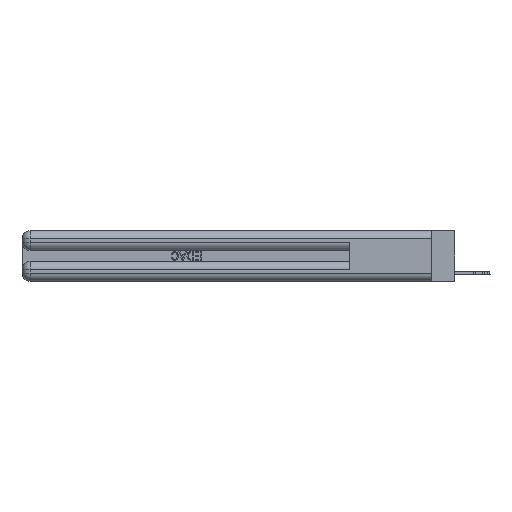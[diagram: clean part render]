
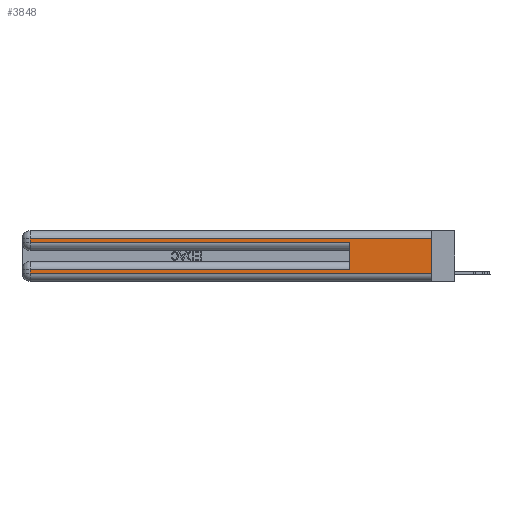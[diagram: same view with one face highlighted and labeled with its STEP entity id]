
A CAD part, left-side view. The second image highlights one B-rep face of the part: STEP entity #3848.
In plain terms, the highlighted planar face has unit normal (-1, 0, 0).
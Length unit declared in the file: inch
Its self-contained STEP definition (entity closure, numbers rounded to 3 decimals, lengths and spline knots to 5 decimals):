
#33 = VECTOR ( 'NONE', #11061, 39.37008 ) ;
#159 = EDGE_CURVE ( 'NONE', #11562, #15059, #29288, .T. ) ;
#877 = DIRECTION ( 'NONE',  ( 1., 0., 0. ) ) ;
#889 = CARTESIAN_POINT ( 'NONE',  ( 0., 0., 0.37 ) ) ;
#2600 = VERTEX_POINT ( 'NONE', #24273 ) ;
#3084 = LINE ( 'NONE', #10879, #33 ) ;
#3848 = ADVANCED_FACE ( 'NONE', ( #14192 ), #19877, .F. ) ;
#4034 = VECTOR ( 'NONE', #12437, 39.37008 ) ;
#4628 = CARTESIAN_POINT ( 'NONE',  ( 0., 0., 0.06 ) ) ;
#4669 = ORIENTED_EDGE ( 'NONE', *, *, #18117, .T. ) ;
#5305 = VECTOR ( 'NONE', #8779, 39.37008 ) ;
#5569 = VECTOR ( 'NONE', #26347, 39.37008 ) ;
#7114 = LINE ( 'NONE', #4628, #4034 ) ;
#7213 = LINE ( 'NONE', #23257, #27163 ) ;
#7887 = EDGE_CURVE ( 'NONE', #25661, #15059, #12553, .T. ) ;
#8728 = DIRECTION ( 'NONE',  ( 0., 0., -1. ) ) ;
#8779 = DIRECTION ( 'NONE',  ( 0., 0., -1. ) ) ;
#9494 = ORIENTED_EDGE ( 'NONE', *, *, #24748, .T. ) ;
#9588 = EDGE_CURVE ( 'NONE', #10633, #13369, #27626, .T. ) ;
#9875 = CARTESIAN_POINT ( 'NONE',  ( 0., 0., 0.285 ) ) ;
#10244 = LINE ( 'NONE', #21129, #5569 ) ;
#10541 = VERTEX_POINT ( 'NONE', #12469 ) ;
#10633 = VERTEX_POINT ( 'NONE', #27107 ) ;
#10879 = CARTESIAN_POINT ( 'NONE',  ( 0., 0., 0.31 ) ) ;
#11061 = DIRECTION ( 'NONE',  ( 0., 1., 0. ) ) ;
#11562 = VERTEX_POINT ( 'NONE', #34271 ) ;
#12437 = DIRECTION ( 'NONE',  ( 0., -1., 0. ) ) ;
#12469 = CARTESIAN_POINT ( 'NONE',  ( 0., 2.94, 0.085 ) ) ;
#12546 = CARTESIAN_POINT ( 'NONE',  ( 0., 2.94, 0.31 ) ) ;
#12553 = LINE ( 'NONE', #9875, #20967 ) ;
#13369 = VERTEX_POINT ( 'NONE', #22543 ) ;
#13451 = CARTESIAN_POINT ( 'NONE',  ( 0., 0.6, 0.145 ) ) ;
#14192 = FACE_OUTER_BOUND ( 'NONE', #31482, .T. ) ;
#14610 = ORIENTED_EDGE ( 'NONE', *, *, #31213, .T. ) ;
#15059 = VERTEX_POINT ( 'NONE', #25050 ) ;
#16038 = ORIENTED_EDGE ( 'NONE', *, *, #159, .F. ) ;
#16811 = CARTESIAN_POINT ( 'NONE',  ( 0., 2.94, 0.285 ) ) ;
#18117 = EDGE_CURVE ( 'NONE', #11562, #10541, #7213, .T. ) ;
#18748 = ORIENTED_EDGE ( 'NONE', *, *, #30964, .T. ) ;
#18758 = VECTOR ( 'NONE', #8728, 39.37008 ) ;
#19245 = LINE ( 'NONE', #32967, #5305 ) ;
#19877 = PLANE ( 'NONE',  #26903 ) ;
#20109 = EDGE_CURVE ( 'NONE', #25873, #25661, #19245, .T. ) ;
#20393 = VECTOR ( 'NONE', #32300, 39.37008 ) ;
#20967 = VECTOR ( 'NONE', #23083, 39.37008 ) ;
#21129 = CARTESIAN_POINT ( 'NONE',  ( 0., 2.94, 0.37 ) ) ;
#22137 = ORIENTED_EDGE ( 'NONE', *, *, #9588, .F. ) ;
#22415 = DIRECTION ( 'NONE',  ( 0., 0., -1. ) ) ;
#22543 = CARTESIAN_POINT ( 'NONE',  ( 0., 0., 0.06 ) ) ;
#23083 = DIRECTION ( 'NONE',  ( 0., -1., 0. ) ) ;
#23257 = CARTESIAN_POINT ( 'NONE',  ( 0., 0., 0.085 ) ) ;
#24273 = CARTESIAN_POINT ( 'NONE',  ( 0., 2.94, 0.06 ) ) ;
#24748 = EDGE_CURVE ( 'NONE', #10541, #2600, #10244, .T. ) ;
#25050 = CARTESIAN_POINT ( 'NONE',  ( 0., 0.6, 0.285 ) ) ;
#25661 = VERTEX_POINT ( 'NONE', #16811 ) ;
#25873 = VERTEX_POINT ( 'NONE', #12546 ) ;
#26347 = DIRECTION ( 'NONE',  ( 0., 0., -1. ) ) ;
#26445 = ORIENTED_EDGE ( 'NONE', *, *, #20109, .T. ) ;
#26903 = AXIS2_PLACEMENT_3D ( 'NONE', #30591, #877, #22415 ) ;
#27107 = CARTESIAN_POINT ( 'NONE',  ( 0., 0., 0.31 ) ) ;
#27163 = VECTOR ( 'NONE', #31576, 39.37008 ) ;
#27626 = LINE ( 'NONE', #889, #18758 ) ;
#29288 = LINE ( 'NONE', #13451, #20393 ) ;
#30591 = CARTESIAN_POINT ( 'NONE',  ( 0., 0., 0.37 ) ) ;
#30964 = EDGE_CURVE ( 'NONE', #10633, #25873, #3084, .T. ) ;
#31213 = EDGE_CURVE ( 'NONE', #2600, #13369, #7114, .T. ) ;
#31482 = EDGE_LOOP ( 'NONE', ( #22137, #18748, #26445, #32158, #16038, #4669, #9494, #14610 ) ) ;
#31576 = DIRECTION ( 'NONE',  ( 0., 1., 0. ) ) ;
#32158 = ORIENTED_EDGE ( 'NONE', *, *, #7887, .T. ) ;
#32300 = DIRECTION ( 'NONE',  ( 0., 0., 1. ) ) ;
#32967 = CARTESIAN_POINT ( 'NONE',  ( 0., 2.94, 0.37 ) ) ;
#34271 = CARTESIAN_POINT ( 'NONE',  ( 0., 0.6, 0.085 ) ) ;
